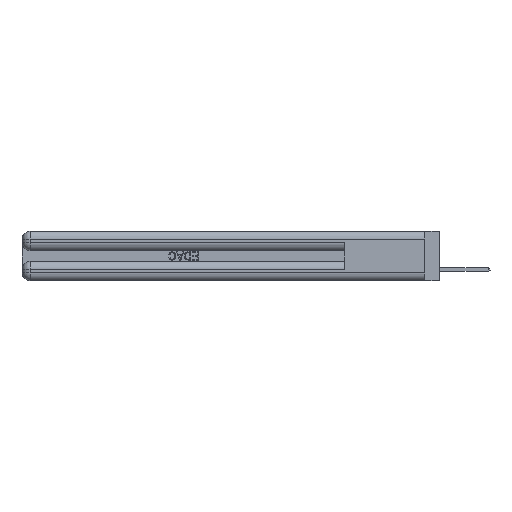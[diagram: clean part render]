
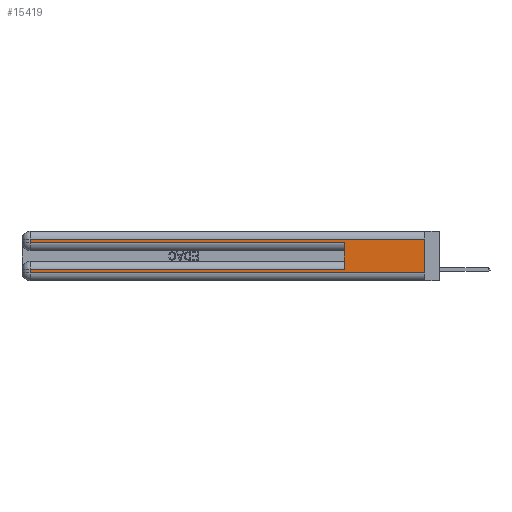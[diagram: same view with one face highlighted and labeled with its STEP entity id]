
A CAD part, left-side view. The second image highlights one B-rep face of the part: STEP entity #15419.
In plain terms, the highlighted planar face has unit normal (-1, 0, 0).
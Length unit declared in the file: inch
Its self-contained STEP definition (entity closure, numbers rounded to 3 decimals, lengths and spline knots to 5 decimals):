
#170 = VECTOR ( 'NONE', #4739, 39.37008 ) ;
#1534 = CARTESIAN_POINT ( 'NONE',  ( 0., 0., 0.31 ) ) ;
#1629 = LINE ( 'NONE', #28260, #25650 ) ;
#2156 = EDGE_CURVE ( 'NONE', #4283, #24253, #3883, .T. ) ;
#2354 = VERTEX_POINT ( 'NONE', #37109 ) ;
#3784 = VECTOR ( 'NONE', #8716, 39.37008 ) ;
#3848 = LINE ( 'NONE', #30410, #11056 ) ;
#3883 = LINE ( 'NONE', #24854, #28491 ) ;
#3920 = VECTOR ( 'NONE', #20311, 39.37008 ) ;
#4025 = EDGE_CURVE ( 'NONE', #26546, #24253, #13821, .T. ) ;
#4283 = VERTEX_POINT ( 'NONE', #33287 ) ;
#4685 = DIRECTION ( 'NONE',  ( 0., 0., -1. ) ) ;
#4739 = DIRECTION ( 'NONE',  ( 0., -1., 0. ) ) ;
#5070 = CARTESIAN_POINT ( 'NONE',  ( 0., 2.94, 0.06 ) ) ;
#5229 = ORIENTED_EDGE ( 'NONE', *, *, #19240, .T. ) ;
#5295 = CARTESIAN_POINT ( 'NONE',  ( 0., 0.6, 0.285 ) ) ;
#5666 = CARTESIAN_POINT ( 'NONE',  ( 0., 0., 0.085 ) ) ;
#6643 = ORIENTED_EDGE ( 'NONE', *, *, #39866, .F. ) ;
#6801 = DIRECTION ( 'NONE',  ( 0., 0., -1. ) ) ;
#8161 = CARTESIAN_POINT ( 'NONE',  ( 0., 0., 0.37 ) ) ;
#8716 = DIRECTION ( 'NONE',  ( 0., 1., 0. ) ) ;
#9298 = LINE ( 'NONE', #25975, #36485 ) ;
#10402 = ORIENTED_EDGE ( 'NONE', *, *, #32188, .T. ) ;
#11056 = VECTOR ( 'NONE', #6801, 39.37008 ) ;
#11131 = AXIS2_PLACEMENT_3D ( 'NONE', #8161, #29660, #4685 ) ;
#11253 = EDGE_CURVE ( 'NONE', #26546, #37301, #19735, .T. ) ;
#12258 = FACE_OUTER_BOUND ( 'NONE', #38050, .T. ) ;
#12458 = CARTESIAN_POINT ( 'NONE',  ( 0., 0.6, 0.145 ) ) ;
#13821 = LINE ( 'NONE', #12458, #34169 ) ;
#14663 = VERTEX_POINT ( 'NONE', #1534 ) ;
#15183 = VERTEX_POINT ( 'NONE', #5070 ) ;
#15419 = ADVANCED_FACE ( 'NONE', ( #12258 ), #17076, .F. ) ;
#15979 = ORIENTED_EDGE ( 'NONE', *, *, #16955, .T. ) ;
#16955 = EDGE_CURVE ( 'NONE', #37301, #15183, #9298, .T. ) ;
#17076 = PLANE ( 'NONE',  #11131 ) ;
#18211 = EDGE_CURVE ( 'NONE', #14663, #2354, #21333, .T. ) ;
#18876 = CARTESIAN_POINT ( 'NONE',  ( 0., 0., 0.06 ) ) ;
#19240 = EDGE_CURVE ( 'NONE', #2354, #4283, #3848, .T. ) ;
#19735 = LINE ( 'NONE', #5666, #3784 ) ;
#19987 = LINE ( 'NONE', #32443, #170 ) ;
#20083 = DIRECTION ( 'NONE',  ( 0., 0., -1. ) ) ;
#20311 = DIRECTION ( 'NONE',  ( 0., 1., 0. ) ) ;
#21333 = LINE ( 'NONE', #29755, #3920 ) ;
#21622 = CARTESIAN_POINT ( 'NONE',  ( 0., 2.94, 0.085 ) ) ;
#24253 = VERTEX_POINT ( 'NONE', #5295 ) ;
#24854 = CARTESIAN_POINT ( 'NONE',  ( 0., 0., 0.285 ) ) ;
#25650 = VECTOR ( 'NONE', #38176, 39.37008 ) ;
#25701 = DIRECTION ( 'NONE',  ( 0., 0., 1. ) ) ;
#25975 = CARTESIAN_POINT ( 'NONE',  ( 0., 2.94, 0.37 ) ) ;
#26546 = VERTEX_POINT ( 'NONE', #26581 ) ;
#26581 = CARTESIAN_POINT ( 'NONE',  ( 0., 0.6, 0.085 ) ) ;
#28152 = ORIENTED_EDGE ( 'NONE', *, *, #4025, .F. ) ;
#28260 = CARTESIAN_POINT ( 'NONE',  ( 0., 0., 0.37 ) ) ;
#28491 = VECTOR ( 'NONE', #38698, 39.37008 ) ;
#28604 = VERTEX_POINT ( 'NONE', #18876 ) ;
#29660 = DIRECTION ( 'NONE',  ( 1., 0., 0. ) ) ;
#29755 = CARTESIAN_POINT ( 'NONE',  ( 0., 0., 0.31 ) ) ;
#30410 = CARTESIAN_POINT ( 'NONE',  ( 0., 2.94, 0.37 ) ) ;
#32188 = EDGE_CURVE ( 'NONE', #15183, #28604, #19987, .T. ) ;
#32443 = CARTESIAN_POINT ( 'NONE',  ( 0., 0., 0.06 ) ) ;
#33287 = CARTESIAN_POINT ( 'NONE',  ( 0., 2.94, 0.285 ) ) ;
#34169 = VECTOR ( 'NONE', #25701, 39.37008 ) ;
#34804 = ORIENTED_EDGE ( 'NONE', *, *, #11253, .T. ) ;
#36027 = ORIENTED_EDGE ( 'NONE', *, *, #2156, .T. ) ;
#36485 = VECTOR ( 'NONE', #20083, 39.37008 ) ;
#36736 = ORIENTED_EDGE ( 'NONE', *, *, #18211, .T. ) ;
#37109 = CARTESIAN_POINT ( 'NONE',  ( 0., 2.94, 0.31 ) ) ;
#37301 = VERTEX_POINT ( 'NONE', #21622 ) ;
#38050 = EDGE_LOOP ( 'NONE', ( #6643, #36736, #5229, #36027, #28152, #34804, #15979, #10402 ) ) ;
#38176 = DIRECTION ( 'NONE',  ( 0., 0., -1. ) ) ;
#38698 = DIRECTION ( 'NONE',  ( 0., -1., 0. ) ) ;
#39866 = EDGE_CURVE ( 'NONE', #14663, #28604, #1629, .T. ) ;
